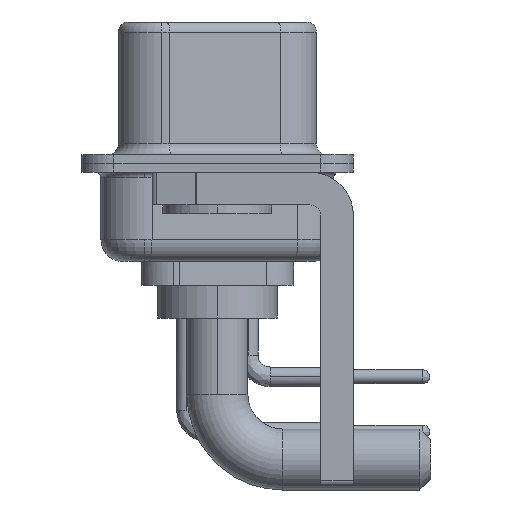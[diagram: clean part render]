
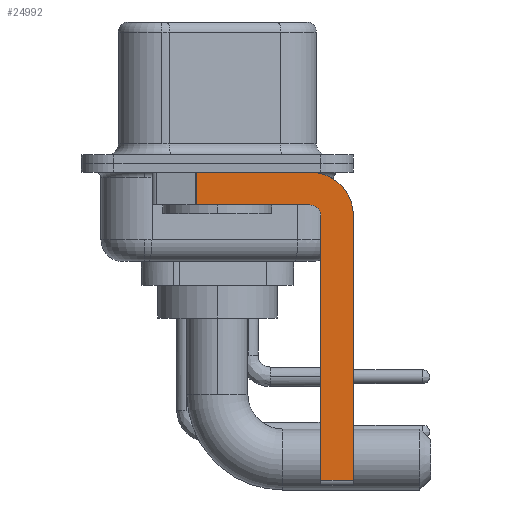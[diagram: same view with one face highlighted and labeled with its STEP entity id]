
A CAD part, left-side view. The second image highlights one B-rep face of the part: STEP entity #24992.
In plain terms, the highlighted planar face has unit normal (-1, 0, 0).
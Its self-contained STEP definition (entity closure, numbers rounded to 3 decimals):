
#298 = EDGE_CURVE ( 'NONE', #3429, #6208, #10048, .T. ) ;
#326 = EDGE_LOOP ( 'NONE', ( #19622, #13947, #22638, #3462, #5252, #2444, #22180, #404 ) ) ;
#404 = ORIENTED_EDGE ( 'NONE', *, *, #298, .F. ) ;
#490 = CARTESIAN_POINT ( 'NONE',  ( -2.9, -4.25, -2.4 ) ) ;
#520 = VECTOR ( 'NONE', #1830, 1000. ) ;
#821 = DIRECTION ( 'NONE',  ( -1., 0., 0. ) ) ;
#1493 = LINE ( 'NONE', #12844, #3637 ) ;
#1830 = DIRECTION ( 'NONE',  ( 0., 1., 0. ) ) ;
#2424 = EDGE_CURVE ( 'NONE', #7244, #3429, #1493, .T. ) ;
#2444 = ORIENTED_EDGE ( 'NONE', *, *, #16118, .T. ) ;
#2710 = VECTOR ( 'NONE', #3403, 1000. ) ;
#3389 = CARTESIAN_POINT ( 'NONE',  ( -2.9, 0.978, -1.9 ) ) ;
#3403 = DIRECTION ( 'NONE',  ( 0., -1., 0. ) ) ;
#3429 = VERTEX_POINT ( 'NONE', #18706 ) ;
#3462 = ORIENTED_EDGE ( 'NONE', *, *, #12940, .F. ) ;
#3637 = VECTOR ( 'NONE', #24959, 1000. ) ;
#4026 = VERTEX_POINT ( 'NONE', #13917 ) ;
#4672 = CARTESIAN_POINT ( 'NONE',  ( -2.9, 0.978, -0.4 ) ) ;
#5252 = ORIENTED_EDGE ( 'NONE', *, *, #12000, .F. ) ;
#5636 = VECTOR ( 'NONE', #18711, 1000. ) ;
#5821 = CARTESIAN_POINT ( 'NONE',  ( -2.9, -4.75, -14.55 ) ) ;
#6208 = VERTEX_POINT ( 'NONE', #10381 ) ;
#6361 = FACE_OUTER_BOUND ( 'NONE', #326, .T. ) ;
#6670 = DIRECTION ( 'NONE',  ( 0., 0., -1. ) ) ;
#7153 = LINE ( 'NONE', #14983, #2710 ) ;
#7166 = CARTESIAN_POINT ( 'NONE',  ( -2.9, 0.978, -1.9 ) ) ;
#7184 = DIRECTION ( 'NONE',  ( 0., 0., 1. ) ) ;
#7244 = VERTEX_POINT ( 'NONE', #4672 ) ;
#8159 = VERTEX_POINT ( 'NONE', #21046 ) ;
#9299 = CARTESIAN_POINT ( 'NONE',  ( -2.9, -4.25, -1.9 ) ) ;
#9897 = AXIS2_PLACEMENT_3D ( 'NONE', #20367, #22446, #15989 ) ;
#10048 = CIRCLE ( 'NONE', #19922, 2. ) ;
#10381 = CARTESIAN_POINT ( 'NONE',  ( -2.9, -6.25, -2.4 ) ) ;
#10509 = LINE ( 'NONE', #24317, #24002 ) ;
#11355 = EDGE_CURVE ( 'NONE', #20127, #19591, #21423, .T. ) ;
#11649 = VECTOR ( 'NONE', #7184, 1000. ) ;
#11939 = EDGE_CURVE ( 'NONE', #6208, #4026, #10509, .T. ) ;
#12000 = EDGE_CURVE ( 'NONE', #25191, #8159, #14759, .T. ) ;
#12480 = DIRECTION ( 'NONE',  ( 1., 0., 0. ) ) ;
#12844 = CARTESIAN_POINT ( 'NONE',  ( -2.9, 3., -0.4 ) ) ;
#12940 = EDGE_CURVE ( 'NONE', #8159, #20127, #20740, .T. ) ;
#12947 = LINE ( 'NONE', #7166, #5636 ) ;
#13917 = CARTESIAN_POINT ( 'NONE',  ( -2.9, -6.25, -14.55 ) ) ;
#13947 = ORIENTED_EDGE ( 'NONE', *, *, #16543, .T. ) ;
#14759 = LINE ( 'NONE', #20815, #11649 ) ;
#14983 = CARTESIAN_POINT ( 'NONE',  ( -2.9, -4.25, -14.55 ) ) ;
#15989 = DIRECTION ( 'NONE',  ( 0., 0., -1. ) ) ;
#16118 = EDGE_CURVE ( 'NONE', #25191, #4026, #7153, .T. ) ;
#16153 = DIRECTION ( 'NONE',  ( 0., 0., 1. ) ) ;
#16543 = EDGE_CURVE ( 'NONE', #7244, #19591, #12947, .T. ) ;
#18175 = PLANE ( 'NONE',  #9897 ) ;
#18706 = CARTESIAN_POINT ( 'NONE',  ( -2.9, -4.25, -0.4 ) ) ;
#18711 = DIRECTION ( 'NONE',  ( 0., 0., -1. ) ) ;
#19558 = CARTESIAN_POINT ( 'NONE',  ( -2.9, -4.25, -1.9 ) ) ;
#19591 = VERTEX_POINT ( 'NONE', #3389 ) ;
#19622 = ORIENTED_EDGE ( 'NONE', *, *, #2424, .F. ) ;
#19922 = AXIS2_PLACEMENT_3D ( 'NONE', #490, #12480, #22143 ) ;
#20127 = VERTEX_POINT ( 'NONE', #19558 ) ;
#20367 = CARTESIAN_POINT ( 'NONE',  ( -2.9, -4.25, -2.4 ) ) ;
#20740 = CIRCLE ( 'NONE', #22807, 0.5 ) ;
#20815 = CARTESIAN_POINT ( 'NONE',  ( -2.9, -4.75, -14.8 ) ) ;
#21046 = CARTESIAN_POINT ( 'NONE',  ( -2.9, -4.75, -2.4 ) ) ;
#21423 = LINE ( 'NONE', #9299, #520 ) ;
#22090 = CARTESIAN_POINT ( 'NONE',  ( -2.9, -4.25, -2.4 ) ) ;
#22143 = DIRECTION ( 'NONE',  ( 0., 0., -1. ) ) ;
#22180 = ORIENTED_EDGE ( 'NONE', *, *, #11939, .F. ) ;
#22446 = DIRECTION ( 'NONE',  ( 1., 0., 0. ) ) ;
#22638 = ORIENTED_EDGE ( 'NONE', *, *, #11355, .F. ) ;
#22807 = AXIS2_PLACEMENT_3D ( 'NONE', #22090, #821, #16153 ) ;
#24002 = VECTOR ( 'NONE', #6670, 1000. ) ;
#24317 = CARTESIAN_POINT ( 'NONE',  ( -2.9, -6.25, -2.4 ) ) ;
#24959 = DIRECTION ( 'NONE',  ( 0., -1., 0. ) ) ;
#24992 = ADVANCED_FACE ( 'NONE', ( #6361 ), #18175, .F. ) ;
#25191 = VERTEX_POINT ( 'NONE', #5821 ) ;
